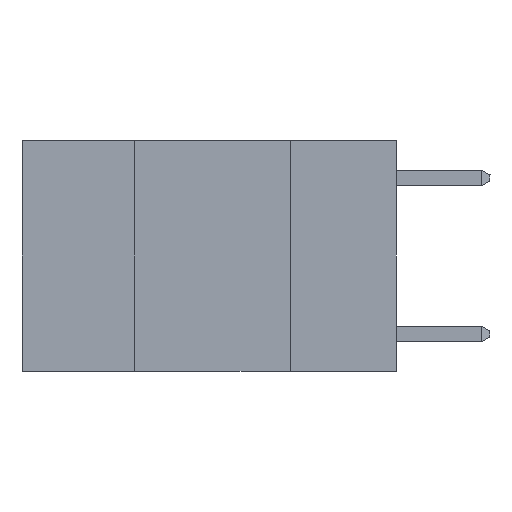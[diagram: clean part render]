
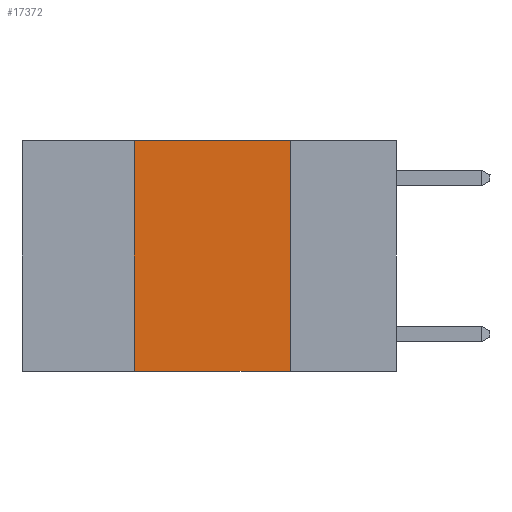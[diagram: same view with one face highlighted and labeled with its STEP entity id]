
A CAD part, left-side view. The second image highlights one B-rep face of the part: STEP entity #17372.
In plain terms, the highlighted planar face has unit normal (-1, 0, 0).
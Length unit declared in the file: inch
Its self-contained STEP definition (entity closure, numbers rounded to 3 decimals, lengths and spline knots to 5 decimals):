
#172 = PLANE ( 'NONE',  #17471 ) ;
#367 = EDGE_CURVE ( 'NONE', #16955, #1002, #1407, .T. ) ;
#395 = EDGE_CURVE ( 'NONE', #11317, #12325, #12811, .T. ) ;
#827 = VECTOR ( 'NONE', #17422, 39.37008 ) ;
#1002 = VERTEX_POINT ( 'NONE', #12418 ) ;
#1407 = LINE ( 'NONE', #12915, #15603 ) ;
#1462 = ORIENTED_EDGE ( 'NONE', *, *, #395, .F. ) ;
#3765 = FACE_OUTER_BOUND ( 'NONE', #13105, .T. ) ;
#4335 = LINE ( 'NONE', #9486, #827 ) ;
#4854 = CARTESIAN_POINT ( 'NONE',  ( 0., 0.42, 0. ) ) ;
#4965 = DIRECTION ( 'NONE',  ( 0., 0., 1. ) ) ;
#6599 = DIRECTION ( 'NONE',  ( 0., 0., -1. ) ) ;
#9207 = CARTESIAN_POINT ( 'NONE',  ( 0., 0.42, 0. ) ) ;
#9440 = VECTOR ( 'NONE', #18868, 39.37008 ) ;
#9486 = CARTESIAN_POINT ( 'NONE',  ( 0., 0.6, -0.37 ) ) ;
#9725 = CARTESIAN_POINT ( 'NONE',  ( 0., 0.17, 0. ) ) ;
#11317 = VERTEX_POINT ( 'NONE', #12062 ) ;
#11915 = VECTOR ( 'NONE', #4965, 39.37008 ) ;
#12062 = CARTESIAN_POINT ( 'NONE',  ( 0., 0.42, -0.37 ) ) ;
#12299 = ORIENTED_EDGE ( 'NONE', *, *, #367, .F. ) ;
#12325 = VERTEX_POINT ( 'NONE', #9207 ) ;
#12418 = CARTESIAN_POINT ( 'NONE',  ( 0., 0.17, -0.37 ) ) ;
#12445 = LINE ( 'NONE', #13991, #9440 ) ;
#12811 = LINE ( 'NONE', #4854, #11915 ) ;
#12915 = CARTESIAN_POINT ( 'NONE',  ( 0., 0.17, 0. ) ) ;
#13081 = CARTESIAN_POINT ( 'NONE',  ( 0., 0.6, 0. ) ) ;
#13105 = EDGE_LOOP ( 'NONE', ( #12299, #13964, #1462, #20551 ) ) ;
#13515 = EDGE_CURVE ( 'NONE', #12325, #16955, #12445, .T. ) ;
#13964 = ORIENTED_EDGE ( 'NONE', *, *, #13515, .F. ) ;
#13991 = CARTESIAN_POINT ( 'NONE',  ( 0., 0.6, 0. ) ) ;
#15603 = VECTOR ( 'NONE', #18948, 39.37008 ) ;
#15896 = EDGE_CURVE ( 'NONE', #11317, #1002, #4335, .T. ) ;
#16955 = VERTEX_POINT ( 'NONE', #9725 ) ;
#17372 = ADVANCED_FACE ( 'NONE', ( #3765 ), #172, .F. ) ;
#17422 = DIRECTION ( 'NONE',  ( 0., -1., 0. ) ) ;
#17471 = AXIS2_PLACEMENT_3D ( 'NONE', #13081, #19318, #6599 ) ;
#18868 = DIRECTION ( 'NONE',  ( 0., -1., 0. ) ) ;
#18948 = DIRECTION ( 'NONE',  ( 0., 0., -1. ) ) ;
#19318 = DIRECTION ( 'NONE',  ( 1., 0., 0. ) ) ;
#20551 = ORIENTED_EDGE ( 'NONE', *, *, #15896, .T. ) ;
